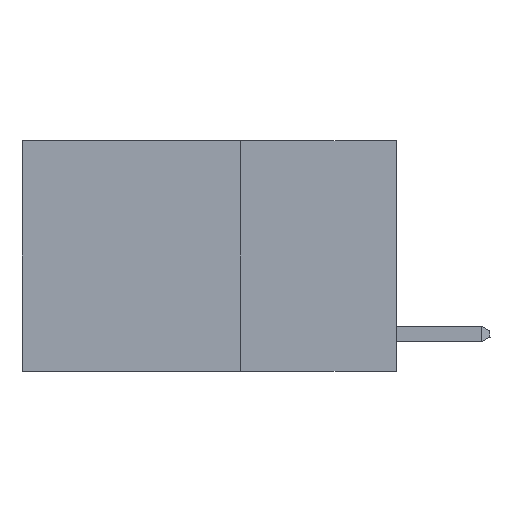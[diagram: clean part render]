
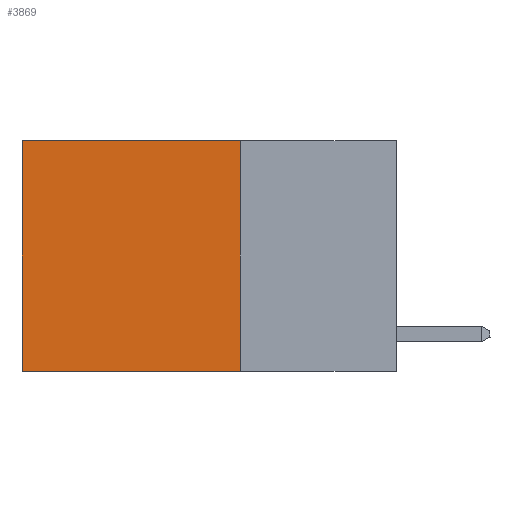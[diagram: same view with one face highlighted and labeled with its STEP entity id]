
A CAD part, left-side view. The second image highlights one B-rep face of the part: STEP entity #3869.
In plain terms, the highlighted planar face has unit normal (-1, 0, 0).
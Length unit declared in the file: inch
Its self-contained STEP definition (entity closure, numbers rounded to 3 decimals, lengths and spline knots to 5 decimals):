
#131 = DIRECTION ( 'NONE',  ( 0., 0., -1. ) ) ;
#375 = ORIENTED_EDGE ( 'NONE', *, *, #8436, .F. ) ;
#500 = EDGE_LOOP ( 'NONE', ( #8079, #375, #12199, #2620 ) ) ;
#544 = DIRECTION ( 'NONE',  ( 0., 0., -1. ) ) ;
#556 = CARTESIAN_POINT ( 'NONE',  ( 0.2625, 0.25, 0. ) ) ;
#1272 = LINE ( 'NONE', #3388, #7070 ) ;
#1390 = VERTEX_POINT ( 'NONE', #5281 ) ;
#1466 = EDGE_CURVE ( 'NONE', #1390, #6211, #7882, .T. ) ;
#2182 = LINE ( 'NONE', #4271, #4563 ) ;
#2620 = ORIENTED_EDGE ( 'NONE', *, *, #1466, .T. ) ;
#2788 = VECTOR ( 'NONE', #12283, 39.37008 ) ;
#2810 = VERTEX_POINT ( 'NONE', #3144 ) ;
#3144 = CARTESIAN_POINT ( 'NONE',  ( 0.2625, 0.6, -0.37 ) ) ;
#3388 = CARTESIAN_POINT ( 'NONE',  ( 0.2625, 0.25, 0. ) ) ;
#3646 = CARTESIAN_POINT ( 'NONE',  ( 0.2625, 0.25, 0. ) ) ;
#3869 = ADVANCED_FACE ( 'NONE', ( #5462 ), #4499, .F. ) ;
#4271 = CARTESIAN_POINT ( 'NONE',  ( 0.2625, 0.6, 0. ) ) ;
#4499 = PLANE ( 'NONE',  #10608 ) ;
#4563 = VECTOR ( 'NONE', #131, 39.37008 ) ;
#5235 = VERTEX_POINT ( 'NONE', #10013 ) ;
#5281 = CARTESIAN_POINT ( 'NONE',  ( 0.2625, 0.25, 0. ) ) ;
#5462 = FACE_OUTER_BOUND ( 'NONE', #500, .T. ) ;
#5540 = DIRECTION ( 'NONE',  ( 0., 0., -1. ) ) ;
#5861 = LINE ( 'NONE', #8000, #2788 ) ;
#6211 = VERTEX_POINT ( 'NONE', #10253 ) ;
#6373 = EDGE_CURVE ( 'NONE', #1390, #5235, #1272, .T. ) ;
#7070 = VECTOR ( 'NONE', #5540, 39.37008 ) ;
#7882 = LINE ( 'NONE', #556, #8363 ) ;
#8000 = CARTESIAN_POINT ( 'NONE',  ( 0.2625, 0.25, -0.37 ) ) ;
#8018 = DIRECTION ( 'NONE',  ( 0., 1., 0. ) ) ;
#8079 = ORIENTED_EDGE ( 'NONE', *, *, #9949, .T. ) ;
#8363 = VECTOR ( 'NONE', #8018, 39.37008 ) ;
#8436 = EDGE_CURVE ( 'NONE', #5235, #2810, #5861, .T. ) ;
#9949 = EDGE_CURVE ( 'NONE', #6211, #2810, #2182, .T. ) ;
#10013 = CARTESIAN_POINT ( 'NONE',  ( 0.2625, 0.25, -0.37 ) ) ;
#10253 = CARTESIAN_POINT ( 'NONE',  ( 0.2625, 0.6, 0. ) ) ;
#10608 = AXIS2_PLACEMENT_3D ( 'NONE', #3646, #13482, #544 ) ;
#12199 = ORIENTED_EDGE ( 'NONE', *, *, #6373, .F. ) ;
#12283 = DIRECTION ( 'NONE',  ( 0., 1., 0. ) ) ;
#13482 = DIRECTION ( 'NONE',  ( 1., 0., 0. ) ) ;
